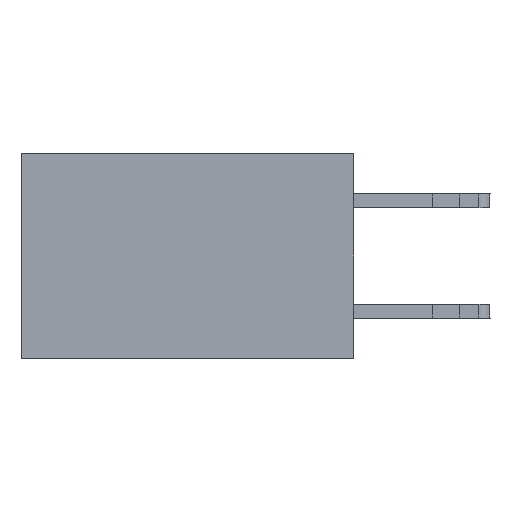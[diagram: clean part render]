
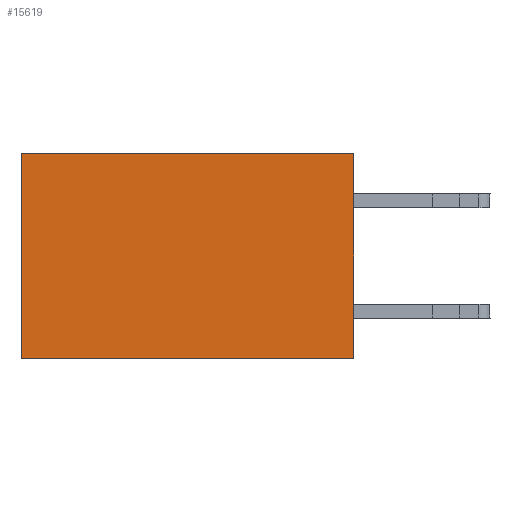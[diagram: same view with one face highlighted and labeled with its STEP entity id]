
A CAD part, left-side view. The second image highlights one B-rep face of the part: STEP entity #15619.
In plain terms, the highlighted planar face has unit normal (-1, 0, 0).
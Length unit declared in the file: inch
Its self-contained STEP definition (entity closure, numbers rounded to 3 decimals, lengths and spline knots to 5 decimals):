
#541 = FACE_OUTER_BOUND ( 'NONE', #34056, .T. ) ;
#2072 = LINE ( 'NONE', #13635, #5531 ) ;
#3432 = VERTEX_POINT ( 'NONE', #27781 ) ;
#3808 = LINE ( 'NONE', #15309, #30698 ) ;
#4396 = DIRECTION ( 'NONE',  ( 0., 0., -1. ) ) ;
#4790 = DIRECTION ( 'NONE',  ( 0., 1., 0. ) ) ;
#5531 = VECTOR ( 'NONE', #4790, 39.37008 ) ;
#5711 = LINE ( 'NONE', #14994, #20456 ) ;
#7028 = DIRECTION ( 'NONE',  ( 0., 0., -1. ) ) ;
#7571 = DIRECTION ( 'NONE',  ( 1., 0., 0. ) ) ;
#9615 = CARTESIAN_POINT ( 'NONE',  ( 0.2875, 0., -0.37 ) ) ;
#10808 = ORIENTED_EDGE ( 'NONE', *, *, #30923, .F. ) ;
#12987 = VECTOR ( 'NONE', #25960, 39.37008 ) ;
#13635 = CARTESIAN_POINT ( 'NONE',  ( 0.2875, 0., 0. ) ) ;
#14730 = EDGE_CURVE ( 'NONE', #18835, #31289, #2072, .T. ) ;
#14745 = CARTESIAN_POINT ( 'NONE',  ( 0.2875, 0., 0. ) ) ;
#14842 = DIRECTION ( 'NONE',  ( 0., 0., -1. ) ) ;
#14994 = CARTESIAN_POINT ( 'NONE',  ( 0.2875, 0.6, 0. ) ) ;
#15309 = CARTESIAN_POINT ( 'NONE',  ( 0.2875, 0., 0. ) ) ;
#15619 = ADVANCED_FACE ( 'NONE', ( #541 ), #28218, .F. ) ;
#16437 = ORIENTED_EDGE ( 'NONE', *, *, #17053, .T. ) ;
#17053 = EDGE_CURVE ( 'NONE', #31289, #3432, #5711, .T. ) ;
#18835 = VERTEX_POINT ( 'NONE', #14745 ) ;
#20456 = VECTOR ( 'NONE', #7028, 39.37008 ) ;
#21521 = AXIS2_PLACEMENT_3D ( 'NONE', #34904, #7571, #4396 ) ;
#24724 = CARTESIAN_POINT ( 'NONE',  ( 0.2875, 0.6, 0. ) ) ;
#24946 = ORIENTED_EDGE ( 'NONE', *, *, #31679, .F. ) ;
#25960 = DIRECTION ( 'NONE',  ( 0., 1., 0. ) ) ;
#26442 = LINE ( 'NONE', #9615, #12987 ) ;
#27781 = CARTESIAN_POINT ( 'NONE',  ( 0.2875, 0.6, -0.37 ) ) ;
#28218 = PLANE ( 'NONE',  #21521 ) ;
#28387 = VERTEX_POINT ( 'NONE', #30948 ) ;
#29748 = ORIENTED_EDGE ( 'NONE', *, *, #14730, .T. ) ;
#30698 = VECTOR ( 'NONE', #14842, 39.37008 ) ;
#30923 = EDGE_CURVE ( 'NONE', #28387, #3432, #26442, .T. ) ;
#30948 = CARTESIAN_POINT ( 'NONE',  ( 0.2875, 0., -0.37 ) ) ;
#31289 = VERTEX_POINT ( 'NONE', #24724 ) ;
#31679 = EDGE_CURVE ( 'NONE', #18835, #28387, #3808, .T. ) ;
#34056 = EDGE_LOOP ( 'NONE', ( #16437, #10808, #24946, #29748 ) ) ;
#34904 = CARTESIAN_POINT ( 'NONE',  ( 0.2875, 0., 0. ) ) ;
